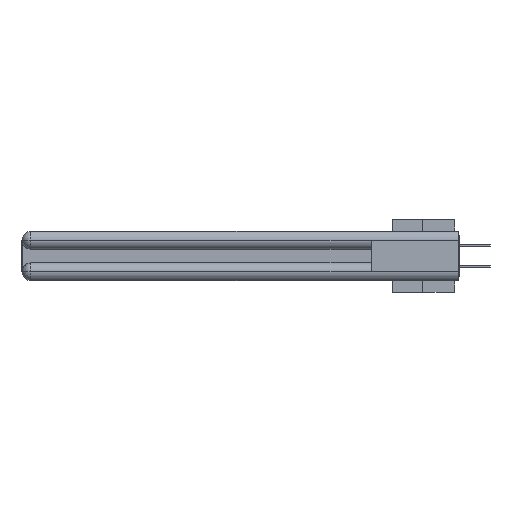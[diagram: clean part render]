
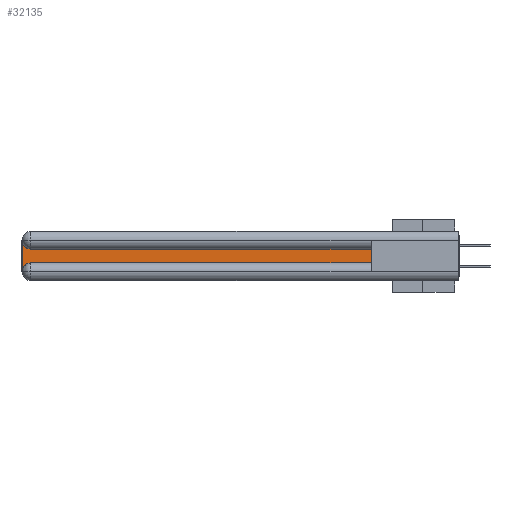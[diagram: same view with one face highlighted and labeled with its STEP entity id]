
A CAD part, left-side view. The second image highlights one B-rep face of the part: STEP entity #32135.
In plain terms, the highlighted planar face has unit normal (-1, 0, 0).
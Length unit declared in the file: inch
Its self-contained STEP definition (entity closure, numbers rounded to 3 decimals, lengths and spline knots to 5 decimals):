
#50 = VECTOR ( 'NONE', #18367, 39.37008 ) ;
#122 = VERTEX_POINT ( 'NONE', #36191 ) ;
#570 = LINE ( 'NONE', #14887, #8893 ) ;
#3778 = CARTESIAN_POINT ( 'NONE',  ( 0.075, 2.94, -0.2775 ) ) ;
#3997 = CARTESIAN_POINT ( 'NONE',  ( 0.075, 0.6, -0.2175 ) ) ;
#5997 = EDGE_CURVE ( 'NONE', #31465, #31143, #22431, .T. ) ;
#7205 = DIRECTION ( 'NONE',  ( 0., 0., -1. ) ) ;
#7570 = AXIS2_PLACEMENT_3D ( 'NONE', #3778, #42662, #7205 ) ;
#8893 = VECTOR ( 'NONE', #39710, 39.37008 ) ;
#10985 = CIRCLE ( 'NONE', #7570, 0.06 ) ;
#11236 = VERTEX_POINT ( 'NONE', #18283 ) ;
#12381 = ORIENTED_EDGE ( 'NONE', *, *, #43129, .T. ) ;
#13201 = ORIENTED_EDGE ( 'NONE', *, *, #5997, .T. ) ;
#14887 = CARTESIAN_POINT ( 'NONE',  ( 0.075, 3., -0.2175 ) ) ;
#16368 = CARTESIAN_POINT ( 'NONE',  ( 0.075, 0.6, -0.2175 ) ) ;
#18283 = CARTESIAN_POINT ( 'NONE',  ( 0.075, 2.94, -0.2175 ) ) ;
#18367 = DIRECTION ( 'NONE',  ( 0., -1., 0. ) ) ;
#18550 = FACE_OUTER_BOUND ( 'NONE', #22676, .T. ) ;
#18824 = AXIS2_PLACEMENT_3D ( 'NONE', #24990, #42927, #25141 ) ;
#19776 = CARTESIAN_POINT ( 'NONE',  ( 0.075, 3., -0.2775 ) ) ;
#20788 = DIRECTION ( 'NONE',  ( 0., 1., 0. ) ) ;
#21080 = CARTESIAN_POINT ( 'NONE',  ( 0.075, 3., -0.0625 ) ) ;
#21543 = PLANE ( 'NONE',  #18824 ) ;
#22431 = LINE ( 'NONE', #16368, #24690 ) ;
#22676 = EDGE_LOOP ( 'NONE', ( #31514, #40968, #28796, #12381, #25394, #13201 ) ) ;
#23422 = LINE ( 'NONE', #42311, #31807 ) ;
#24155 = DIRECTION ( 'NONE',  ( 0., 0., -1. ) ) ;
#24690 = VECTOR ( 'NONE', #44304, 39.37008 ) ;
#24990 = CARTESIAN_POINT ( 'NONE',  ( 0.075, 3., -0.1225 ) ) ;
#25141 = DIRECTION ( 'NONE',  ( 0., 0., -1. ) ) ;
#25288 = CARTESIAN_POINT ( 'NONE',  ( 0.075, 0.6, -0.2175 ) ) ;
#25394 = ORIENTED_EDGE ( 'NONE', *, *, #33593, .T. ) ;
#27515 = EDGE_CURVE ( 'NONE', #122, #43464, #28519, .T. ) ;
#27747 = CARTESIAN_POINT ( 'NONE',  ( 0.075, 2.94, -0.0625 ) ) ;
#28519 = CIRCLE ( 'NONE', #33607, 0.06 ) ;
#28796 = ORIENTED_EDGE ( 'NONE', *, *, #34099, .T. ) ;
#31143 = VERTEX_POINT ( 'NONE', #40631 ) ;
#31465 = VERTEX_POINT ( 'NONE', #25288 ) ;
#31514 = ORIENTED_EDGE ( 'NONE', *, *, #34139, .T. ) ;
#31807 = VECTOR ( 'NONE', #20788, 39.37008 ) ;
#32135 = ADVANCED_FACE ( 'NONE', ( #18550 ), #21543, .F. ) ;
#33593 = EDGE_CURVE ( 'NONE', #11236, #31465, #38980, .T. ) ;
#33607 = AXIS2_PLACEMENT_3D ( 'NONE', #27747, #41796, #24155 ) ;
#34099 = EDGE_CURVE ( 'NONE', #43464, #44997, #570, .T. ) ;
#34139 = EDGE_CURVE ( 'NONE', #31143, #122, #23422, .T. ) ;
#36191 = CARTESIAN_POINT ( 'NONE',  ( 0.075, 2.94, -0.1225 ) ) ;
#38980 = LINE ( 'NONE', #3997, #50 ) ;
#39710 = DIRECTION ( 'NONE',  ( 0., 0., -1. ) ) ;
#40631 = CARTESIAN_POINT ( 'NONE',  ( 0.075, 0.6, -0.1225 ) ) ;
#40968 = ORIENTED_EDGE ( 'NONE', *, *, #27515, .T. ) ;
#41796 = DIRECTION ( 'NONE',  ( 1., 0., 0. ) ) ;
#42311 = CARTESIAN_POINT ( 'NONE',  ( 0.075, 0.6, -0.1225 ) ) ;
#42662 = DIRECTION ( 'NONE',  ( 1., 0., 0. ) ) ;
#42927 = DIRECTION ( 'NONE',  ( 1., 0., 0. ) ) ;
#43129 = EDGE_CURVE ( 'NONE', #44997, #11236, #10985, .T. ) ;
#43464 = VERTEX_POINT ( 'NONE', #21080 ) ;
#44304 = DIRECTION ( 'NONE',  ( 0., 0., 1. ) ) ;
#44997 = VERTEX_POINT ( 'NONE', #19776 ) ;
